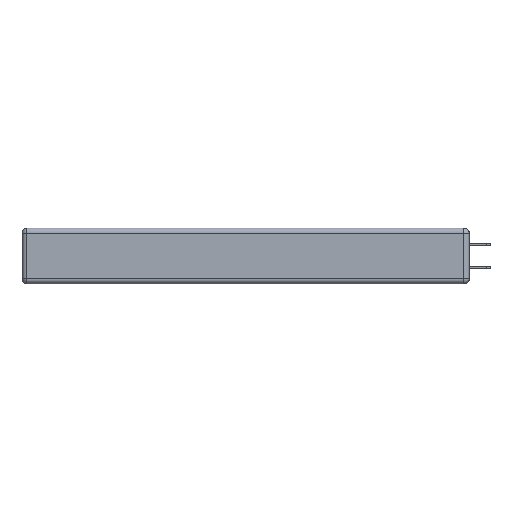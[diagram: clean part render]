
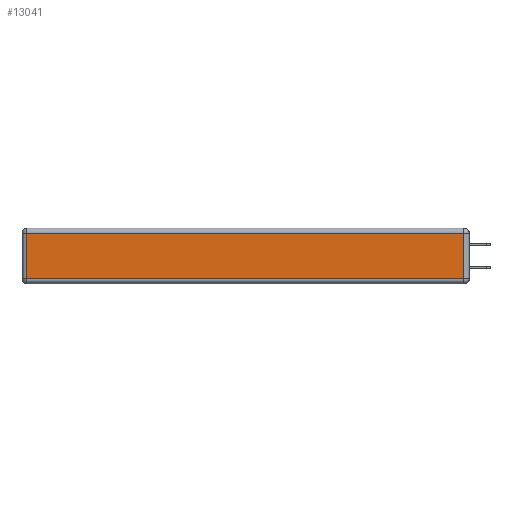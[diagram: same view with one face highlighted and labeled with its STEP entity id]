
A CAD part, left-side view. The second image highlights one B-rep face of the part: STEP entity #13041.
In plain terms, the highlighted planar face has unit normal (-1, 0, 0).
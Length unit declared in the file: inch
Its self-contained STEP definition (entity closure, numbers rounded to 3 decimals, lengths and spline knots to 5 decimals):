
#1062 = CARTESIAN_POINT ( 'NONE',  ( 0., 0., -0.313 ) ) ;
#1157 = DIRECTION ( 'NONE',  ( -1., 0., 0. ) ) ;
#1164 = EDGE_CURVE ( 'NONE', #15000, #4326, #9074, .T. ) ;
#1472 = VERTEX_POINT ( 'NONE', #6181 ) ;
#1805 = EDGE_CURVE ( 'NONE', #8988, #15000, #8209, .T. ) ;
#2394 = CARTESIAN_POINT ( 'NONE',  ( 0., 2.75, -0.03 ) ) ;
#2721 = DIRECTION ( 'NONE',  ( 0., 0., 1. ) ) ;
#3462 = VECTOR ( 'NONE', #6681, 39.37008 ) ;
#3759 = ORIENTED_EDGE ( 'NONE', *, *, #1164, .T. ) ;
#4326 = VERTEX_POINT ( 'NONE', #12759 ) ;
#4800 = ORIENTED_EDGE ( 'NONE', *, *, #1805, .T. ) ;
#4974 = CARTESIAN_POINT ( 'NONE',  ( 0., 2.72, -0.313 ) ) ;
#5143 = EDGE_LOOP ( 'NONE', ( #4800, #3759, #10264, #10929 ) ) ;
#5494 = DIRECTION ( 'NONE',  ( 0., 1., 0. ) ) ;
#5897 = LINE ( 'NONE', #2394, #9552 ) ;
#6181 = CARTESIAN_POINT ( 'NONE',  ( 0., 2.72, -0.03 ) ) ;
#6681 = DIRECTION ( 'NONE',  ( 0., 0., -1. ) ) ;
#7015 = LINE ( 'NONE', #16030, #3462 ) ;
#8209 = LINE ( 'NONE', #1062, #12397 ) ;
#8988 = VERTEX_POINT ( 'NONE', #4974 ) ;
#9074 = LINE ( 'NONE', #16200, #12208 ) ;
#9552 = VECTOR ( 'NONE', #5494, 39.37008 ) ;
#9995 = EDGE_CURVE ( 'NONE', #1472, #8988, #7015, .T. ) ;
#10099 = FACE_OUTER_BOUND ( 'NONE', #5143, .T. ) ;
#10264 = ORIENTED_EDGE ( 'NONE', *, *, #16338, .T. ) ;
#10799 = PLANE ( 'NONE',  #16473 ) ;
#10929 = ORIENTED_EDGE ( 'NONE', *, *, #9995, .T. ) ;
#12208 = VECTOR ( 'NONE', #2721, 39.37008 ) ;
#12227 = CARTESIAN_POINT ( 'NONE',  ( 0., 0.03, -0.313 ) ) ;
#12397 = VECTOR ( 'NONE', #16136, 39.37008 ) ;
#12759 = CARTESIAN_POINT ( 'NONE',  ( 0., 0.03, -0.03 ) ) ;
#13041 = ADVANCED_FACE ( 'NONE', ( #10099 ), #10799, .T. ) ;
#13302 = DIRECTION ( 'NONE',  ( 0., 0., 1. ) ) ;
#15000 = VERTEX_POINT ( 'NONE', #12227 ) ;
#16030 = CARTESIAN_POINT ( 'NONE',  ( 0., 2.72, -0.343 ) ) ;
#16136 = DIRECTION ( 'NONE',  ( 0., -1., 0. ) ) ;
#16200 = CARTESIAN_POINT ( 'NONE',  ( 0., 0.03, -0.343 ) ) ;
#16338 = EDGE_CURVE ( 'NONE', #4326, #1472, #5897, .T. ) ;
#16473 = AXIS2_PLACEMENT_3D ( 'NONE', #17306, #1157, #13302 ) ;
#17306 = CARTESIAN_POINT ( 'NONE',  ( 0., 0., -0.343 ) ) ;
